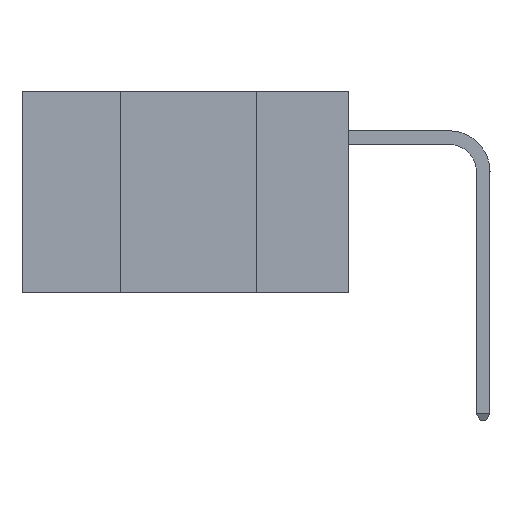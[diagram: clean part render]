
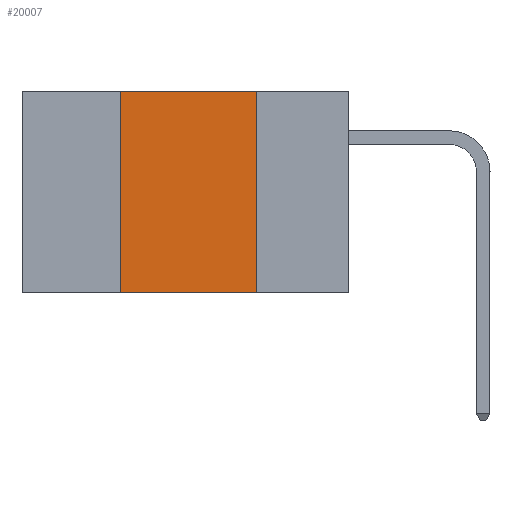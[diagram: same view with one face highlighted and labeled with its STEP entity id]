
A CAD part, left-side view. The second image highlights one B-rep face of the part: STEP entity #20007.
In plain terms, the highlighted planar face has unit normal (-1, 0, 0).
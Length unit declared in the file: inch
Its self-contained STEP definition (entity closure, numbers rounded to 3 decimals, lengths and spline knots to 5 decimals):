
#2060 = VERTEX_POINT ( 'NONE', #32459 ) ;
#2932 = LINE ( 'NONE', #23953, #12048 ) ;
#3184 = CARTESIAN_POINT ( 'NONE',  ( 0., 0.6, -0.37 ) ) ;
#5466 = CARTESIAN_POINT ( 'NONE',  ( 0., 0.17, 0. ) ) ;
#6923 = CARTESIAN_POINT ( 'NONE',  ( 0., 0.6, 0. ) ) ;
#7816 = ORIENTED_EDGE ( 'NONE', *, *, #22035, .F. ) ;
#8911 = CARTESIAN_POINT ( 'NONE',  ( 0., 0.42, 0. ) ) ;
#9504 = LINE ( 'NONE', #6923, #31130 ) ;
#10720 = VECTOR ( 'NONE', #14707, 39.37008 ) ;
#11342 = PLANE ( 'NONE',  #14148 ) ;
#11557 = VERTEX_POINT ( 'NONE', #8911 ) ;
#12048 = VECTOR ( 'NONE', #21360, 39.37008 ) ;
#14148 = AXIS2_PLACEMENT_3D ( 'NONE', #29803, #21842, #29454 ) ;
#14707 = DIRECTION ( 'NONE',  ( 0., -1., 0. ) ) ;
#15150 = DIRECTION ( 'NONE',  ( 0., 0., 1. ) ) ;
#15185 = EDGE_CURVE ( 'NONE', #23791, #11557, #22909, .T. ) ;
#16278 = LINE ( 'NONE', #3184, #10720 ) ;
#17409 = DIRECTION ( 'NONE',  ( 0., -1., 0. ) ) ;
#17603 = ORIENTED_EDGE ( 'NONE', *, *, #15185, .F. ) ;
#18388 = VECTOR ( 'NONE', #15150, 39.37008 ) ;
#18440 = CARTESIAN_POINT ( 'NONE',  ( 0., 0.42, -0.37 ) ) ;
#20007 = ADVANCED_FACE ( 'NONE', ( #32050 ), #11342, .F. ) ;
#21360 = DIRECTION ( 'NONE',  ( 0., 0., -1. ) ) ;
#21733 = EDGE_LOOP ( 'NONE', ( #7816, #31368, #17603, #30949 ) ) ;
#21842 = DIRECTION ( 'NONE',  ( 1., 0., 0. ) ) ;
#22035 = EDGE_CURVE ( 'NONE', #24665, #2060, #2932, .T. ) ;
#22909 = LINE ( 'NONE', #33452, #18388 ) ;
#23791 = VERTEX_POINT ( 'NONE', #18440 ) ;
#23953 = CARTESIAN_POINT ( 'NONE',  ( 0., 0.17, 0. ) ) ;
#24665 = VERTEX_POINT ( 'NONE', #5466 ) ;
#26569 = EDGE_CURVE ( 'NONE', #23791, #2060, #16278, .T. ) ;
#27125 = EDGE_CURVE ( 'NONE', #11557, #24665, #9504, .T. ) ;
#29454 = DIRECTION ( 'NONE',  ( 0., 0., -1. ) ) ;
#29803 = CARTESIAN_POINT ( 'NONE',  ( 0., 0.6, 0. ) ) ;
#30949 = ORIENTED_EDGE ( 'NONE', *, *, #26569, .T. ) ;
#31130 = VECTOR ( 'NONE', #17409, 39.37008 ) ;
#31368 = ORIENTED_EDGE ( 'NONE', *, *, #27125, .F. ) ;
#32050 = FACE_OUTER_BOUND ( 'NONE', #21733, .T. ) ;
#32459 = CARTESIAN_POINT ( 'NONE',  ( 0., 0.17, -0.37 ) ) ;
#33452 = CARTESIAN_POINT ( 'NONE',  ( 0., 0.42, 0. ) ) ;
